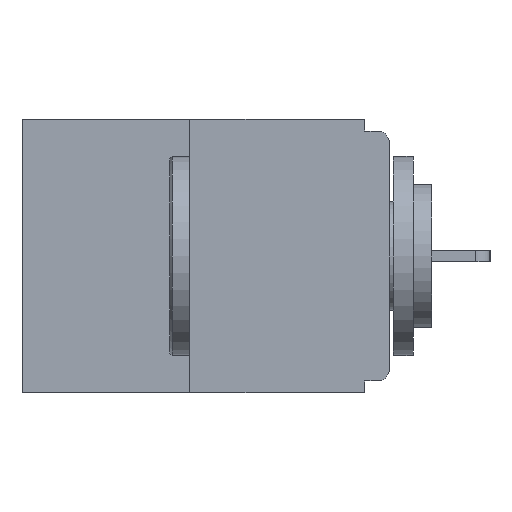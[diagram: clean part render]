
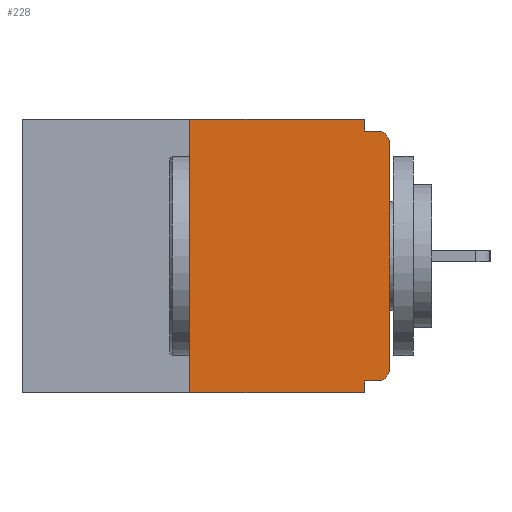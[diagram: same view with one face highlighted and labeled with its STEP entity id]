
A CAD part, left-side view. The second image highlights one B-rep face of the part: STEP entity #228.
In plain terms, the highlighted planar face has unit normal (-1, 0, 0).
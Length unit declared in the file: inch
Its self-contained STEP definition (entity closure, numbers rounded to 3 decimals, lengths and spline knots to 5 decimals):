
#120 = LINE ( 'NONE', #7946, #13915 ) ;
#228 = ADVANCED_FACE ( 'NONE', ( #18859 ), #7958, .F. ) ;
#283 = CIRCLE ( 'NONE', #11654, 0.015 ) ;
#465 = LINE ( 'NONE', #16033, #13979 ) ;
#551 = CARTESIAN_POINT ( 'NONE',  ( 0., 0., -0.328 ) ) ;
#873 = DIRECTION ( 'NONE',  ( 0., 0., -1. ) ) ;
#997 = LINE ( 'NONE', #15136, #9543 ) ;
#1131 = AXIS2_PLACEMENT_3D ( 'NONE', #15899, #17334, #5094 ) ;
#1438 = CARTESIAN_POINT ( 'NONE',  ( 0., 0.25, 0. ) ) ;
#1516 = VERTEX_POINT ( 'NONE', #14480 ) ;
#1685 = DIRECTION ( 'NONE',  ( -1., 0., 0. ) ) ;
#1813 = ORIENTED_EDGE ( 'NONE', *, *, #15704, .F. ) ;
#2385 = CARTESIAN_POINT ( 'NONE',  ( 0., 0., -0.313 ) ) ;
#2497 = CARTESIAN_POINT ( 'NONE',  ( 0., 0.015, -0.015 ) ) ;
#2670 = VERTEX_POINT ( 'NONE', #2497 ) ;
#2703 = LINE ( 'NONE', #14820, #18508 ) ;
#2969 = LINE ( 'NONE', #1438, #9440 ) ;
#3176 = EDGE_CURVE ( 'NONE', #11037, #2670, #120, .T. ) ;
#3683 = VECTOR ( 'NONE', #10038, 39.37008 ) ;
#3816 = VERTEX_POINT ( 'NONE', #12595 ) ;
#4874 = ORIENTED_EDGE ( 'NONE', *, *, #13325, .T. ) ;
#5094 = DIRECTION ( 'NONE',  ( 0., 0., -1. ) ) ;
#5137 = LINE ( 'NONE', #7061, #16352 ) ;
#5178 = VERTEX_POINT ( 'NONE', #7295 ) ;
#5655 = VERTEX_POINT ( 'NONE', #14733 ) ;
#5743 = DIRECTION ( 'NONE',  ( 0., -1., 0. ) ) ;
#6011 = DIRECTION ( 'NONE',  ( 0., -1., 0. ) ) ;
#6519 = ORIENTED_EDGE ( 'NONE', *, *, #7855, .T. ) ;
#6732 = ORIENTED_EDGE ( 'NONE', *, *, #3176, .F. ) ;
#6738 = DIRECTION ( 'NONE',  ( -1., 0., 0. ) ) ;
#7061 = CARTESIAN_POINT ( 'NONE',  ( 0., 0.46, -0.343 ) ) ;
#7285 = ORIENTED_EDGE ( 'NONE', *, *, #10861, .F. ) ;
#7295 = CARTESIAN_POINT ( 'NONE',  ( 0., 0.25, 0. ) ) ;
#7516 = VERTEX_POINT ( 'NONE', #15563 ) ;
#7633 = DIRECTION ( 'NONE',  ( 0., 0., 1. ) ) ;
#7855 = EDGE_CURVE ( 'NONE', #12914, #7930, #283, .T. ) ;
#7863 = EDGE_CURVE ( 'NONE', #12914, #12060, #19288, .T. ) ;
#7930 = VERTEX_POINT ( 'NONE', #2385 ) ;
#7946 = CARTESIAN_POINT ( 'NONE',  ( 0., 0., -0.015 ) ) ;
#7958 = PLANE ( 'NONE',  #1131 ) ;
#7986 = CARTESIAN_POINT ( 'NONE',  ( 0., 0.015, -0.03 ) ) ;
#8184 = DIRECTION ( 'NONE',  ( 0., 1., 0. ) ) ;
#8378 = DIRECTION ( 'NONE',  ( 0., 0., -1. ) ) ;
#8643 = ORIENTED_EDGE ( 'NONE', *, *, #13210, .T. ) ;
#8735 = ORIENTED_EDGE ( 'NONE', *, *, #19776, .F. ) ;
#9440 = VECTOR ( 'NONE', #7633, 39.37008 ) ;
#9543 = VECTOR ( 'NONE', #5743, 39.37008 ) ;
#9556 = AXIS2_PLACEMENT_3D ( 'NONE', #7986, #1685, #16968 ) ;
#9831 = DIRECTION ( 'NONE',  ( 0., 0., -1. ) ) ;
#10038 = DIRECTION ( 'NONE',  ( 0., 0., 1. ) ) ;
#10045 = VECTOR ( 'NONE', #8184, 39.37008 ) ;
#10620 = ORIENTED_EDGE ( 'NONE', *, *, #7863, .F. ) ;
#10861 = EDGE_CURVE ( 'NONE', #3816, #5178, #2969, .T. ) ;
#11037 = VERTEX_POINT ( 'NONE', #12517 ) ;
#11175 = EDGE_LOOP ( 'NONE', ( #1813, #7285, #8643, #8735, #10620, #6519, #4874, #13908, #6732, #16721 ) ) ;
#11654 = AXIS2_PLACEMENT_3D ( 'NONE', #12955, #6738, #8378 ) ;
#12060 = VERTEX_POINT ( 'NONE', #19767 ) ;
#12517 = CARTESIAN_POINT ( 'NONE',  ( 0., 0.031, -0.015 ) ) ;
#12595 = CARTESIAN_POINT ( 'NONE',  ( 0., 0.25, -0.343 ) ) ;
#12802 = CIRCLE ( 'NONE', #9556, 0.015 ) ;
#12914 = VERTEX_POINT ( 'NONE', #20119 ) ;
#12955 = CARTESIAN_POINT ( 'NONE',  ( 0., 0.015, -0.313 ) ) ;
#13210 = EDGE_CURVE ( 'NONE', #3816, #1516, #5137, .T. ) ;
#13325 = EDGE_CURVE ( 'NONE', #7930, #7516, #16351, .T. ) ;
#13908 = ORIENTED_EDGE ( 'NONE', *, *, #15868, .T. ) ;
#13915 = VECTOR ( 'NONE', #6011, 39.37008 ) ;
#13979 = VECTOR ( 'NONE', #9831, 39.37008 ) ;
#14480 = CARTESIAN_POINT ( 'NONE',  ( 0., 0.031, -0.343 ) ) ;
#14733 = CARTESIAN_POINT ( 'NONE',  ( 0., 0.031, 0. ) ) ;
#14820 = CARTESIAN_POINT ( 'NONE',  ( 0., 0.031, -0.343 ) ) ;
#15136 = CARTESIAN_POINT ( 'NONE',  ( 0., 0.46, 0. ) ) ;
#15563 = CARTESIAN_POINT ( 'NONE',  ( 0., 0., -0.03 ) ) ;
#15704 = EDGE_CURVE ( 'NONE', #5178, #5655, #997, .T. ) ;
#15868 = EDGE_CURVE ( 'NONE', #7516, #2670, #12802, .T. ) ;
#15899 = CARTESIAN_POINT ( 'NONE',  ( 0., 0.46, 0. ) ) ;
#16033 = CARTESIAN_POINT ( 'NONE',  ( 0., 0.031, 0. ) ) ;
#16351 = LINE ( 'NONE', #19101, #3683 ) ;
#16352 = VECTOR ( 'NONE', #19508, 39.37008 ) ;
#16721 = ORIENTED_EDGE ( 'NONE', *, *, #19584, .F. ) ;
#16968 = DIRECTION ( 'NONE',  ( 0., 0., -1. ) ) ;
#17334 = DIRECTION ( 'NONE',  ( 1., 0., 0. ) ) ;
#18508 = VECTOR ( 'NONE', #873, 39.37008 ) ;
#18859 = FACE_OUTER_BOUND ( 'NONE', #11175, .T. ) ;
#19101 = CARTESIAN_POINT ( 'NONE',  ( 0., 0., 0. ) ) ;
#19288 = LINE ( 'NONE', #551, #10045 ) ;
#19508 = DIRECTION ( 'NONE',  ( 0., -1., 0. ) ) ;
#19584 = EDGE_CURVE ( 'NONE', #5655, #11037, #465, .T. ) ;
#19767 = CARTESIAN_POINT ( 'NONE',  ( 0., 0.031, -0.328 ) ) ;
#19776 = EDGE_CURVE ( 'NONE', #12060, #1516, #2703, .T. ) ;
#20119 = CARTESIAN_POINT ( 'NONE',  ( 0., 0.015, -0.328 ) ) ;
